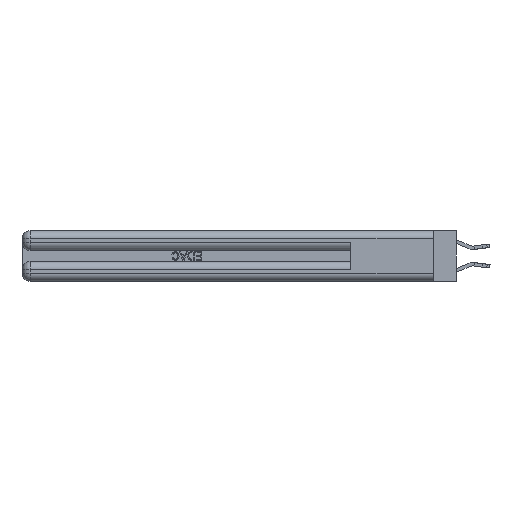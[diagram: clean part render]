
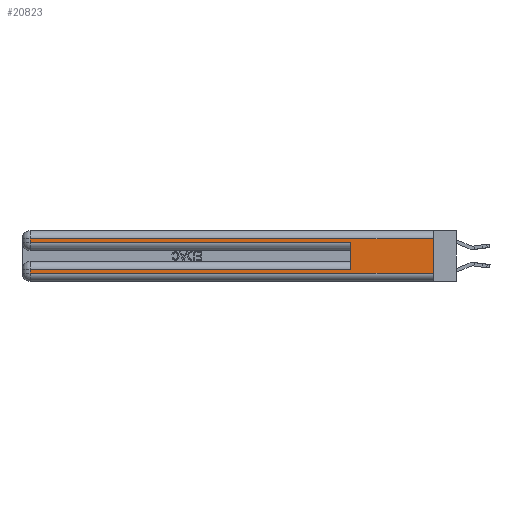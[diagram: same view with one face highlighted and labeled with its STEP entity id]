
A CAD part, left-side view. The second image highlights one B-rep face of the part: STEP entity #20823.
In plain terms, the highlighted planar face has unit normal (-1, 0, 0).
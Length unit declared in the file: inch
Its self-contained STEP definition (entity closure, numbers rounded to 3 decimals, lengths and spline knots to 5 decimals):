
#510 = VERTEX_POINT ( 'NONE', #27171 ) ;
#2167 = LINE ( 'NONE', #6020, #14663 ) ;
#2251 = VECTOR ( 'NONE', #28272, 39.37008 ) ;
#2597 = CARTESIAN_POINT ( 'NONE',  ( 0., 2.94, 0.37 ) ) ;
#2613 = VECTOR ( 'NONE', #14311, 39.37008 ) ;
#2685 = VECTOR ( 'NONE', #23809, 39.37008 ) ;
#3235 = EDGE_CURVE ( 'NONE', #24999, #17968, #26935, .T. ) ;
#3405 = PLANE ( 'NONE',  #13362 ) ;
#3629 = EDGE_CURVE ( 'NONE', #17968, #25088, #4036, .T. ) ;
#3666 = EDGE_CURVE ( 'NONE', #13388, #510, #28355, .T. ) ;
#4036 = LINE ( 'NONE', #21170, #15821 ) ;
#4830 = DIRECTION ( 'NONE',  ( 0., -1., 0. ) ) ;
#5316 = CARTESIAN_POINT ( 'NONE',  ( 0., 0.6, 0.145 ) ) ;
#6020 = CARTESIAN_POINT ( 'NONE',  ( 0., 0., 0.37 ) ) ;
#6978 = CARTESIAN_POINT ( 'NONE',  ( 0., 0., 0.31 ) ) ;
#7165 = CARTESIAN_POINT ( 'NONE',  ( 0., 0.6, 0.285 ) ) ;
#7560 = CARTESIAN_POINT ( 'NONE',  ( 0., 2.94, 0.06 ) ) ;
#7662 = EDGE_CURVE ( 'NONE', #30479, #14857, #25607, .T. ) ;
#8086 = CARTESIAN_POINT ( 'NONE',  ( 0., 2.94, 0.085 ) ) ;
#8442 = EDGE_CURVE ( 'NONE', #30479, #25088, #12329, .T. ) ;
#9579 = VECTOR ( 'NONE', #4830, 39.37008 ) ;
#10493 = DIRECTION ( 'NONE',  ( 0., 0., -1. ) ) ;
#10976 = EDGE_CURVE ( 'NONE', #14857, #13388, #14002, .T. ) ;
#11430 = CARTESIAN_POINT ( 'NONE',  ( 0., 2.94, 0.285 ) ) ;
#11584 = VECTOR ( 'NONE', #17032, 39.37008 ) ;
#11711 = EDGE_CURVE ( 'NONE', #21188, #24999, #16656, .T. ) ;
#11802 = CARTESIAN_POINT ( 'NONE',  ( 0., 2.94, 0.37 ) ) ;
#11833 = DIRECTION ( 'NONE',  ( 0., -1., 0. ) ) ;
#12329 = LINE ( 'NONE', #5316, #11584 ) ;
#12885 = ORIENTED_EDGE ( 'NONE', *, *, #3666, .T. ) ;
#13362 = AXIS2_PLACEMENT_3D ( 'NONE', #15140, #24600, #10493 ) ;
#13388 = VERTEX_POINT ( 'NONE', #7560 ) ;
#14002 = LINE ( 'NONE', #11802, #2251 ) ;
#14023 = CARTESIAN_POINT ( 'NONE',  ( 0., 0., 0.31 ) ) ;
#14311 = DIRECTION ( 'NONE',  ( 0., 0., -1. ) ) ;
#14409 = DIRECTION ( 'NONE',  ( 0., 1., 0. ) ) ;
#14663 = VECTOR ( 'NONE', #22480, 39.37008 ) ;
#14857 = VERTEX_POINT ( 'NONE', #8086 ) ;
#15004 = EDGE_CURVE ( 'NONE', #21188, #510, #2167, .T. ) ;
#15140 = CARTESIAN_POINT ( 'NONE',  ( 0., 0., 0.37 ) ) ;
#15349 = ORIENTED_EDGE ( 'NONE', *, *, #3629, .T. ) ;
#15821 = VECTOR ( 'NONE', #11833, 39.37008 ) ;
#15856 = FACE_OUTER_BOUND ( 'NONE', #21315, .T. ) ;
#16656 = LINE ( 'NONE', #14023, #2685 ) ;
#17032 = DIRECTION ( 'NONE',  ( 0., 0., 1. ) ) ;
#17515 = CARTESIAN_POINT ( 'NONE',  ( 0., 0.6, 0.085 ) ) ;
#17968 = VERTEX_POINT ( 'NONE', #11430 ) ;
#18419 = ORIENTED_EDGE ( 'NONE', *, *, #10976, .T. ) ;
#19123 = CARTESIAN_POINT ( 'NONE',  ( 0., 0., 0.085 ) ) ;
#19307 = VECTOR ( 'NONE', #14409, 39.37008 ) ;
#19662 = ORIENTED_EDGE ( 'NONE', *, *, #7662, .T. ) ;
#20142 = ORIENTED_EDGE ( 'NONE', *, *, #3235, .T. ) ;
#20823 = ADVANCED_FACE ( 'NONE', ( #15856 ), #3405, .F. ) ;
#21129 = ORIENTED_EDGE ( 'NONE', *, *, #11711, .T. ) ;
#21170 = CARTESIAN_POINT ( 'NONE',  ( 0., 0., 0.285 ) ) ;
#21188 = VERTEX_POINT ( 'NONE', #6978 ) ;
#21263 = CARTESIAN_POINT ( 'NONE',  ( 0., 0., 0.06 ) ) ;
#21315 = EDGE_LOOP ( 'NONE', ( #22210, #21129, #20142, #15349, #24534, #19662, #18419, #12885 ) ) ;
#22210 = ORIENTED_EDGE ( 'NONE', *, *, #15004, .F. ) ;
#22480 = DIRECTION ( 'NONE',  ( 0., 0., -1. ) ) ;
#23809 = DIRECTION ( 'NONE',  ( 0., 1., 0. ) ) ;
#24534 = ORIENTED_EDGE ( 'NONE', *, *, #8442, .F. ) ;
#24600 = DIRECTION ( 'NONE',  ( 1., 0., 0. ) ) ;
#24999 = VERTEX_POINT ( 'NONE', #25404 ) ;
#25088 = VERTEX_POINT ( 'NONE', #7165 ) ;
#25404 = CARTESIAN_POINT ( 'NONE',  ( 0., 2.94, 0.31 ) ) ;
#25607 = LINE ( 'NONE', #19123, #19307 ) ;
#26935 = LINE ( 'NONE', #2597, #2613 ) ;
#27171 = CARTESIAN_POINT ( 'NONE',  ( 0., 0., 0.06 ) ) ;
#28272 = DIRECTION ( 'NONE',  ( 0., 0., -1. ) ) ;
#28355 = LINE ( 'NONE', #21263, #9579 ) ;
#30479 = VERTEX_POINT ( 'NONE', #17515 ) ;
